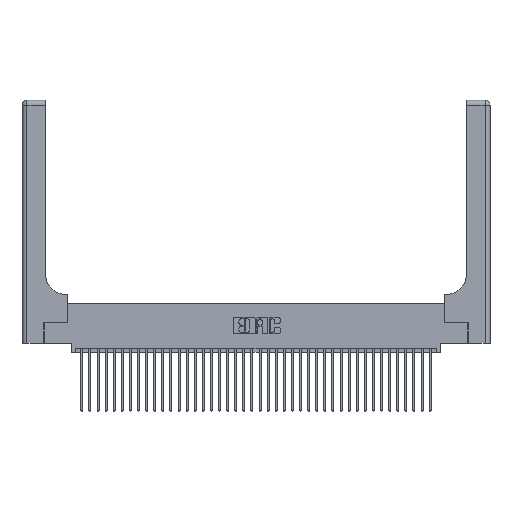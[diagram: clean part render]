
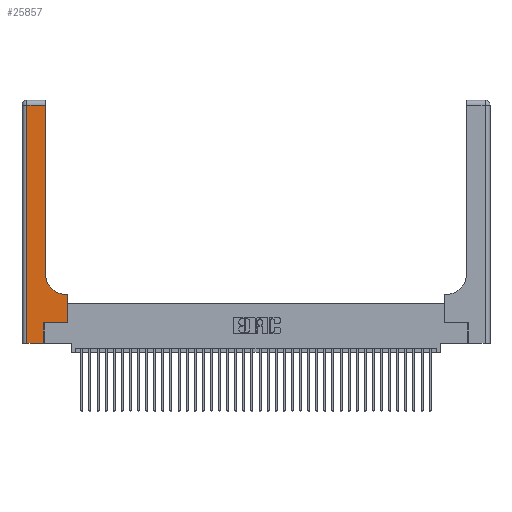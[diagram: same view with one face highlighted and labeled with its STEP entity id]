
A CAD part, top view. The second image highlights one B-rep face of the part: STEP entity #25857.
In plain terms, the highlighted planar face has unit normal (0, 0, 1).
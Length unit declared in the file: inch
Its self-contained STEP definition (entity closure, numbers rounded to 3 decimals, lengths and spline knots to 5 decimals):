
#1017 = EDGE_CURVE ( 'NONE', #4782, #16009, #35689, .T. ) ;
#1584 = CARTESIAN_POINT ( 'NONE',  ( 0., 3., 0.37 ) ) ;
#2022 = DIRECTION ( 'NONE',  ( 1., 0., 0. ) ) ;
#2808 = EDGE_CURVE ( 'NONE', #15453, #37804, #16527, .T. ) ;
#3624 = CARTESIAN_POINT ( 'NONE',  ( 0.5585, 0.25, 0.37 ) ) ;
#3833 = VECTOR ( 'NONE', #10790, 39.37008 ) ;
#4782 = VERTEX_POINT ( 'NONE', #18323 ) ;
#5180 = EDGE_CURVE ( 'NONE', #36717, #22569, #26743, .T. ) ;
#5483 = LINE ( 'NONE', #32048, #20897 ) ;
#5505 = VECTOR ( 'NONE', #6797, 39.37008 ) ;
#5905 = CARTESIAN_POINT ( 'NONE',  ( 0.5585, 0.25, 0.37 ) ) ;
#6244 = EDGE_CURVE ( 'NONE', #16009, #36311, #5483, .T. ) ;
#6458 = CARTESIAN_POINT ( 'NONE',  ( 0.2915, 2.94, 0.37 ) ) ;
#6680 = DIRECTION ( 'NONE',  ( 0., 1., 0. ) ) ;
#6797 = DIRECTION ( 'NONE',  ( 1., 0., 0. ) ) ;
#7699 = CARTESIAN_POINT ( 'NONE',  ( 0.269, 0., 0.37 ) ) ;
#7740 = PLANE ( 'NONE',  #11802 ) ;
#8626 = DIRECTION ( 'NONE',  ( -1., 0., 0. ) ) ;
#10165 = FACE_OUTER_BOUND ( 'NONE', #11228, .T. ) ;
#10620 = ORIENTED_EDGE ( 'NONE', *, *, #5180, .T. ) ;
#10790 = DIRECTION ( 'NONE',  ( 0., 1., 0. ) ) ;
#10830 = DIRECTION ( 'NONE',  ( -1., 0., 0. ) ) ;
#11223 = VECTOR ( 'NONE', #6680, 39.37008 ) ;
#11228 = EDGE_LOOP ( 'NONE', ( #28333, #21843, #26189, #24828, #22496, #18326, #14294, #22932, #10620 ) ) ;
#11295 = VECTOR ( 'NONE', #13137, 39.37008 ) ;
#11802 = AXIS2_PLACEMENT_3D ( 'NONE', #1584, #29178, #10830 ) ;
#12012 = VERTEX_POINT ( 'NONE', #6458 ) ;
#13137 = DIRECTION ( 'NONE',  ( 0., -1., 0. ) ) ;
#13552 = CARTESIAN_POINT ( 'NONE',  ( 0.06, 0., 0.37 ) ) ;
#14294 = ORIENTED_EDGE ( 'NONE', *, *, #2808, .T. ) ;
#14627 = LINE ( 'NONE', #39244, #29931 ) ;
#14804 = EDGE_CURVE ( 'NONE', #22569, #12012, #26558, .T. ) ;
#15170 = CARTESIAN_POINT ( 'NONE',  ( 0.269, 0.25, 0.37 ) ) ;
#15453 = VERTEX_POINT ( 'NONE', #5905 ) ;
#15638 = LINE ( 'NONE', #34347, #5505 ) ;
#16009 = VERTEX_POINT ( 'NONE', #13552 ) ;
#16527 = LINE ( 'NONE', #3624, #11223 ) ;
#16638 = EDGE_CURVE ( 'NONE', #36311, #35969, #29233, .T. ) ;
#18323 = CARTESIAN_POINT ( 'NONE',  ( 0.06, 2.94, 0.37 ) ) ;
#18326 = ORIENTED_EDGE ( 'NONE', *, *, #36162, .T. ) ;
#18426 = VECTOR ( 'NONE', #36723, 39.37008 ) ;
#20066 = VECTOR ( 'NONE', #8626, 39.37008 ) ;
#20418 = DIRECTION ( 'NONE',  ( 0., 0., -1. ) ) ;
#20526 = CARTESIAN_POINT ( 'NONE',  ( 0.5585, 0.6, 0.37 ) ) ;
#20897 = VECTOR ( 'NONE', #38023, 39.37008 ) ;
#21843 = ORIENTED_EDGE ( 'NONE', *, *, #36605, .T. ) ;
#22240 = CARTESIAN_POINT ( 'NONE',  ( 0.269, 0., 0.37 ) ) ;
#22381 = CARTESIAN_POINT ( 'NONE',  ( 0.06, 3., 0.37 ) ) ;
#22496 = ORIENTED_EDGE ( 'NONE', *, *, #16638, .T. ) ;
#22569 = VERTEX_POINT ( 'NONE', #31716 ) ;
#22932 = ORIENTED_EDGE ( 'NONE', *, *, #34775, .T. ) ;
#24100 = DIRECTION ( 'NONE',  ( -1., 0., 0. ) ) ;
#24828 = ORIENTED_EDGE ( 'NONE', *, *, #6244, .T. ) ;
#25857 = ADVANCED_FACE ( 'NONE', ( #10165 ), #7740, .F. ) ;
#26189 = ORIENTED_EDGE ( 'NONE', *, *, #1017, .T. ) ;
#26558 = LINE ( 'NONE', #27569, #18426 ) ;
#26743 = CIRCLE ( 'NONE', #38896, 0.25 ) ;
#27569 = CARTESIAN_POINT ( 'NONE',  ( 0.2915, 3., 0.37 ) ) ;
#28181 = LINE ( 'NONE', #39121, #20066 ) ;
#28333 = ORIENTED_EDGE ( 'NONE', *, *, #14804, .T. ) ;
#29178 = DIRECTION ( 'NONE',  ( 0., 0., -1. ) ) ;
#29233 = LINE ( 'NONE', #7699, #3833 ) ;
#29931 = VECTOR ( 'NONE', #24100, 39.37008 ) ;
#30586 = CARTESIAN_POINT ( 'NONE',  ( 0.5415, 0.6, 0.37 ) ) ;
#31716 = CARTESIAN_POINT ( 'NONE',  ( 0.2915, 0.85, 0.37 ) ) ;
#32048 = CARTESIAN_POINT ( 'NONE',  ( 0., 0., 0.37 ) ) ;
#34347 = CARTESIAN_POINT ( 'NONE',  ( 0.269, 0.25, 0.37 ) ) ;
#34775 = EDGE_CURVE ( 'NONE', #37804, #36717, #28181, .T. ) ;
#35689 = LINE ( 'NONE', #22381, #11295 ) ;
#35969 = VERTEX_POINT ( 'NONE', #15170 ) ;
#36162 = EDGE_CURVE ( 'NONE', #35969, #15453, #15638, .T. ) ;
#36311 = VERTEX_POINT ( 'NONE', #22240 ) ;
#36605 = EDGE_CURVE ( 'NONE', #12012, #4782, #14627, .T. ) ;
#36717 = VERTEX_POINT ( 'NONE', #30586 ) ;
#36723 = DIRECTION ( 'NONE',  ( 0., 1., 0. ) ) ;
#37804 = VERTEX_POINT ( 'NONE', #20526 ) ;
#38023 = DIRECTION ( 'NONE',  ( 1., 0., 0. ) ) ;
#38635 = CARTESIAN_POINT ( 'NONE',  ( 0.5415, 0.85, 0.37 ) ) ;
#38896 = AXIS2_PLACEMENT_3D ( 'NONE', #38635, #20418, #2022 ) ;
#39121 = CARTESIAN_POINT ( 'NONE',  ( 0.2915, 0.6, 0.37 ) ) ;
#39244 = CARTESIAN_POINT ( 'NONE',  ( 0., 2.94, 0.37 ) ) ;
